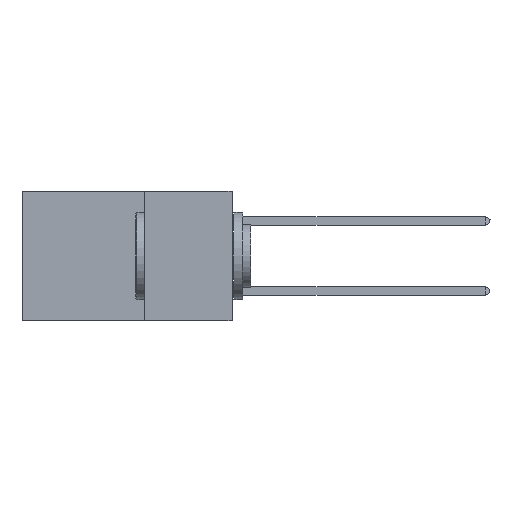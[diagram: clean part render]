
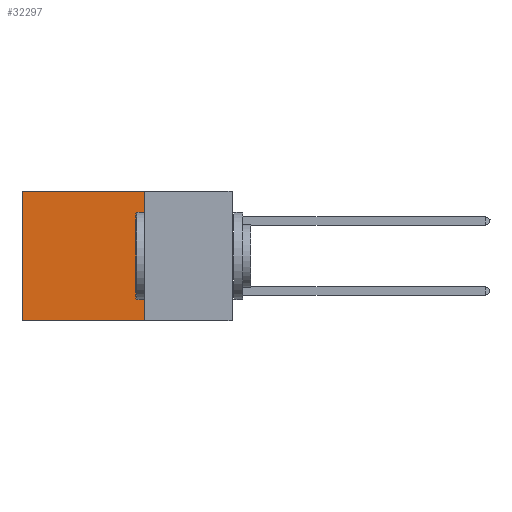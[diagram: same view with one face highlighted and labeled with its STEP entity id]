
A CAD part, left-side view. The second image highlights one B-rep face of the part: STEP entity #32297.
In plain terms, the highlighted planar face has unit normal (-1, 0, 0).
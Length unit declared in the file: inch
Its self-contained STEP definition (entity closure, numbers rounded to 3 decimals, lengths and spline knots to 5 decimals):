
#1816 = LINE ( 'NONE', #33080, #8085 ) ;
#2506 = DIRECTION ( 'NONE',  ( 1., 0., 0. ) ) ;
#2720 = DIRECTION ( 'NONE',  ( 0., 0., -1. ) ) ;
#3008 = EDGE_CURVE ( 'NONE', #33325, #19699, #19800, .T. ) ;
#4390 = EDGE_CURVE ( 'NONE', #21089, #30380, #21754, .T. ) ;
#6255 = VECTOR ( 'NONE', #30023, 39.37008 ) ;
#7581 = VECTOR ( 'NONE', #26768, 39.37008 ) ;
#7750 = CARTESIAN_POINT ( 'NONE',  ( 0.2875, 0.25, -0.37 ) ) ;
#8085 = VECTOR ( 'NONE', #14781, 39.37008 ) ;
#9983 = FACE_OUTER_BOUND ( 'NONE', #33671, .T. ) ;
#13149 = PLANE ( 'NONE',  #22269 ) ;
#13207 = CARTESIAN_POINT ( 'NONE',  ( 0.2875, 0.6, 0. ) ) ;
#14781 = DIRECTION ( 'NONE',  ( 0., 1., 0. ) ) ;
#15622 = CARTESIAN_POINT ( 'NONE',  ( 0.2875, 0.25, 0. ) ) ;
#16052 = CARTESIAN_POINT ( 'NONE',  ( 0.2875, 0.6, 0. ) ) ;
#16535 = ORIENTED_EDGE ( 'NONE', *, *, #4390, .F. ) ;
#16931 = CARTESIAN_POINT ( 'NONE',  ( 0.2875, 0.25, 0. ) ) ;
#18149 = VECTOR ( 'NONE', #2720, 39.37008 ) ;
#18492 = EDGE_CURVE ( 'NONE', #21089, #33325, #21272, .T. ) ;
#18859 = CARTESIAN_POINT ( 'NONE',  ( 0.2875, 0.25, 0. ) ) ;
#19155 = CARTESIAN_POINT ( 'NONE',  ( 0.2875, 0.6, -0.37 ) ) ;
#19699 = VERTEX_POINT ( 'NONE', #19155 ) ;
#19800 = LINE ( 'NONE', #16052, #18149 ) ;
#21089 = VERTEX_POINT ( 'NONE', #32606 ) ;
#21158 = DIRECTION ( 'NONE',  ( 0., 0., -1. ) ) ;
#21272 = LINE ( 'NONE', #16931, #6255 ) ;
#21754 = LINE ( 'NONE', #18859, #7581 ) ;
#22269 = AXIS2_PLACEMENT_3D ( 'NONE', #15622, #2506, #21158 ) ;
#22554 = EDGE_CURVE ( 'NONE', #30380, #19699, #1816, .T. ) ;
#26768 = DIRECTION ( 'NONE',  ( 0., 0., -1. ) ) ;
#28613 = ORIENTED_EDGE ( 'NONE', *, *, #22554, .F. ) ;
#29154 = ORIENTED_EDGE ( 'NONE', *, *, #3008, .T. ) ;
#30023 = DIRECTION ( 'NONE',  ( 0., 1., 0. ) ) ;
#30380 = VERTEX_POINT ( 'NONE', #7750 ) ;
#31227 = ORIENTED_EDGE ( 'NONE', *, *, #18492, .T. ) ;
#32297 = ADVANCED_FACE ( 'NONE', ( #9983 ), #13149, .F. ) ;
#32606 = CARTESIAN_POINT ( 'NONE',  ( 0.2875, 0.25, 0. ) ) ;
#33080 = CARTESIAN_POINT ( 'NONE',  ( 0.2875, 0.25, -0.37 ) ) ;
#33325 = VERTEX_POINT ( 'NONE', #13207 ) ;
#33671 = EDGE_LOOP ( 'NONE', ( #29154, #28613, #16535, #31227 ) ) ;
